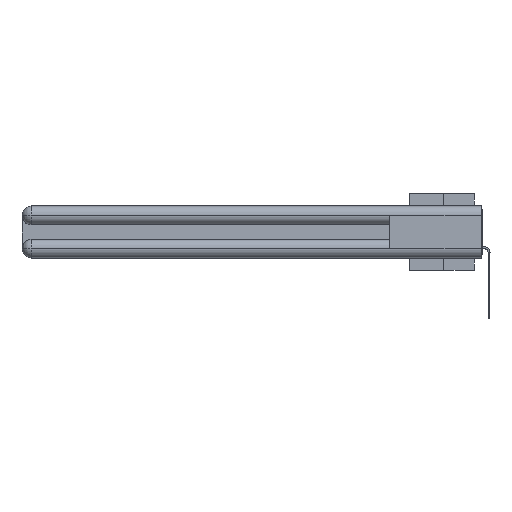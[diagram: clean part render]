
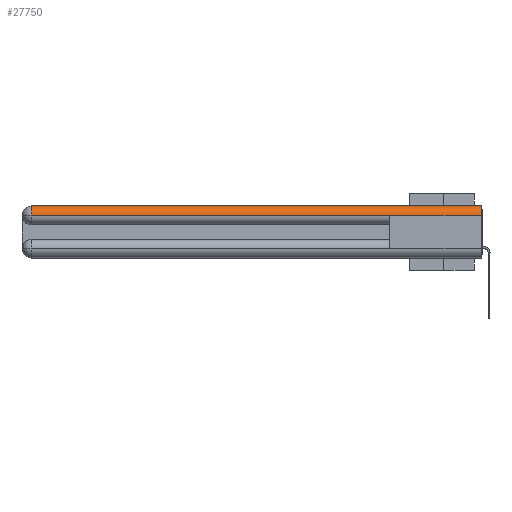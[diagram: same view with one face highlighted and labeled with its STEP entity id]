
A CAD part, left-side view. The second image highlights one B-rep face of the part: STEP entity #27750.
In plain terms, the highlighted cylindrical face has radius 1.562 mm (diameter 3.124 mm), a partial arc.
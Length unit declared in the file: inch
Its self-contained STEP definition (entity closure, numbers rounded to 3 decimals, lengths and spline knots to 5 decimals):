
#811 = DIRECTION ( 'NONE',  ( 1., 0., 0. ) ) ;
#945 = CARTESIAN_POINT ( 'NONE',  ( 0., 3., -0.0615 ) ) ;
#1101 = LINE ( 'NONE', #24917, #6263 ) ;
#1458 = EDGE_CURVE ( 'NONE', #33451, #22132, #8949, .T. ) ;
#1946 = VECTOR ( 'NONE', #6184, 39.37008 ) ;
#2244 = CIRCLE ( 'NONE', #23900, 0.0615 ) ;
#2558 = ORIENTED_EDGE ( 'NONE', *, *, #18553, .T. ) ;
#2911 = VECTOR ( 'NONE', #29825, 39.37008 ) ;
#3463 = CARTESIAN_POINT ( 'NONE',  ( 0.0615, 0., -0.0615 ) ) ;
#5156 = ORIENTED_EDGE ( 'NONE', *, *, #1458, .F. ) ;
#6184 = DIRECTION ( 'NONE',  ( 0., -1., 0. ) ) ;
#6263 = VECTOR ( 'NONE', #22328, 39.37008 ) ;
#6547 = EDGE_CURVE ( 'NONE', #22132, #11111, #15102, .T. ) ;
#7508 = VERTEX_POINT ( 'NONE', #32885 ) ;
#8270 = EDGE_CURVE ( 'NONE', #11111, #7508, #21487, .T. ) ;
#8949 = LINE ( 'NONE', #27574, #1946 ) ;
#11111 = VERTEX_POINT ( 'NONE', #21244 ) ;
#11569 = CARTESIAN_POINT ( 'NONE',  ( 0., 2.94, -0.0615 ) ) ;
#11636 = DIRECTION ( 'NONE',  ( 0., 1., 0. ) ) ;
#12255 = VERTEX_POINT ( 'NONE', #11569 ) ;
#12738 = EDGE_CURVE ( 'NONE', #33451, #12255, #2244, .T. ) ;
#14329 = CARTESIAN_POINT ( 'NONE',  ( 0.0615, 2.94, -0.0615 ) ) ;
#15102 = CIRCLE ( 'NONE', #27859, 0.0615 ) ;
#16305 = DIRECTION ( 'NONE',  ( 0., -1., 0. ) ) ;
#16767 = DIRECTION ( 'NONE',  ( 0., -1., 0. ) ) ;
#17285 = DIRECTION ( 'NONE',  ( 0., 0., 1. ) ) ;
#17976 = ORIENTED_EDGE ( 'NONE', *, *, #12738, .T. ) ;
#18553 = EDGE_CURVE ( 'NONE', #12255, #7508, #1101, .T. ) ;
#20007 = AXIS2_PLACEMENT_3D ( 'NONE', #3463, #11636, #32518 ) ;
#20637 = CARTESIAN_POINT ( 'NONE',  ( 0.0615, 0., 0. ) ) ;
#21034 = ORIENTED_EDGE ( 'NONE', *, *, #8270, .F. ) ;
#21244 = CARTESIAN_POINT ( 'NONE',  ( 0., 0., -0.0615 ) ) ;
#21487 = LINE ( 'NONE', #945, #2911 ) ;
#22132 = VERTEX_POINT ( 'NONE', #20637 ) ;
#22328 = DIRECTION ( 'NONE',  ( 0., -1., 0. ) ) ;
#23900 = AXIS2_PLACEMENT_3D ( 'NONE', #14329, #16767, #17285 ) ;
#24917 = CARTESIAN_POINT ( 'NONE',  ( 0., 3., -0.0615 ) ) ;
#26088 = CARTESIAN_POINT ( 'NONE',  ( 0.0615, 2.94, 0. ) ) ;
#27574 = CARTESIAN_POINT ( 'NONE',  ( 0.0615, 0., 0. ) ) ;
#27750 = ADVANCED_FACE ( 'NONE', ( #33024 ), #30067, .T. ) ;
#27859 = AXIS2_PLACEMENT_3D ( 'NONE', #30015, #16305, #811 ) ;
#28667 = ORIENTED_EDGE ( 'NONE', *, *, #6547, .F. ) ;
#29254 = EDGE_LOOP ( 'NONE', ( #5156, #17976, #2558, #21034, #28667 ) ) ;
#29825 = DIRECTION ( 'NONE',  ( 0., 1., 0. ) ) ;
#30015 = CARTESIAN_POINT ( 'NONE',  ( 0.0615, 0., -0.0615 ) ) ;
#30067 = CYLINDRICAL_SURFACE ( 'NONE', #20007, 0.0615 ) ;
#32518 = DIRECTION ( 'NONE',  ( 0., 0., 1. ) ) ;
#32885 = CARTESIAN_POINT ( 'NONE',  ( 0., 0.6, -0.0615 ) ) ;
#33024 = FACE_OUTER_BOUND ( 'NONE', #29254, .T. ) ;
#33451 = VERTEX_POINT ( 'NONE', #26088 ) ;
